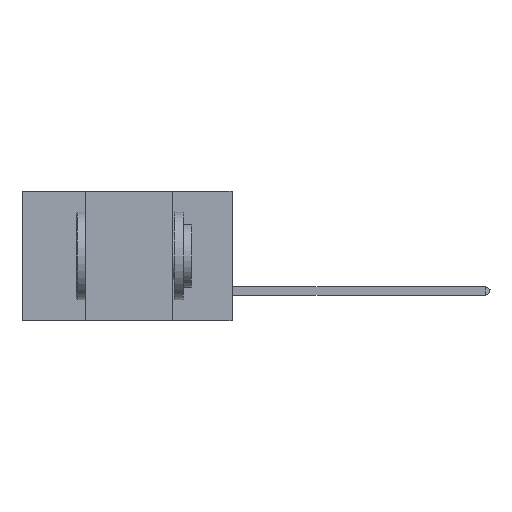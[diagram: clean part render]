
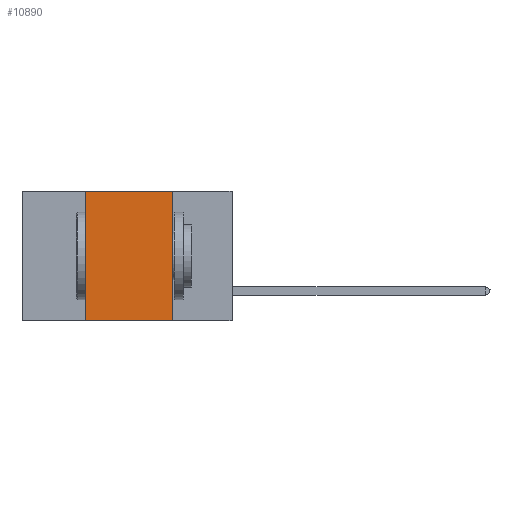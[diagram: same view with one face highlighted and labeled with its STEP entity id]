
A CAD part, left-side view. The second image highlights one B-rep face of the part: STEP entity #10890.
In plain terms, the highlighted planar face has unit normal (-1, 0, 0).
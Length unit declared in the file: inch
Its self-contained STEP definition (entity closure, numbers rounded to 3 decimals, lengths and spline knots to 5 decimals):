
#165 = DIRECTION ( 'NONE',  ( 0., 0., 1. ) ) ;
#483 = AXIS2_PLACEMENT_3D ( 'NONE', #10939, #2225, #4361 ) ;
#484 = CARTESIAN_POINT ( 'NONE',  ( 0., 0.6, -0.37 ) ) ;
#1360 = VERTEX_POINT ( 'NONE', #13789 ) ;
#1533 = VERTEX_POINT ( 'NONE', #3362 ) ;
#1584 = EDGE_LOOP ( 'NONE', ( #12478, #13533, #6326, #3112 ) ) ;
#1849 = VERTEX_POINT ( 'NONE', #3999 ) ;
#1929 = DIRECTION ( 'NONE',  ( 0., 0., -1. ) ) ;
#2007 = CARTESIAN_POINT ( 'NONE',  ( 0., 0.42, 0. ) ) ;
#2194 = VECTOR ( 'NONE', #11205, 39.37008 ) ;
#2225 = DIRECTION ( 'NONE',  ( 1., 0., 0. ) ) ;
#2637 = FACE_OUTER_BOUND ( 'NONE', #1584, .T. ) ;
#2908 = CARTESIAN_POINT ( 'NONE',  ( 0., 0.17, 0. ) ) ;
#2979 = LINE ( 'NONE', #9774, #13731 ) ;
#3112 = ORIENTED_EDGE ( 'NONE', *, *, #5513, .T. ) ;
#3362 = CARTESIAN_POINT ( 'NONE',  ( 0., 0.17, 0. ) ) ;
#3999 = CARTESIAN_POINT ( 'NONE',  ( 0., 0.42, -0.37 ) ) ;
#4361 = DIRECTION ( 'NONE',  ( 0., 0., -1. ) ) ;
#4731 = VERTEX_POINT ( 'NONE', #2007 ) ;
#5513 = EDGE_CURVE ( 'NONE', #1849, #1360, #10258, .T. ) ;
#6317 = VECTOR ( 'NONE', #1929, 39.37008 ) ;
#6326 = ORIENTED_EDGE ( 'NONE', *, *, #7049, .F. ) ;
#6571 = PLANE ( 'NONE',  #483 ) ;
#7049 = EDGE_CURVE ( 'NONE', #1849, #4731, #2979, .T. ) ;
#8129 = EDGE_CURVE ( 'NONE', #4731, #1533, #12055, .T. ) ;
#9686 = VECTOR ( 'NONE', #10607, 39.37008 ) ;
#9774 = CARTESIAN_POINT ( 'NONE',  ( 0., 0.42, 0. ) ) ;
#9877 = LINE ( 'NONE', #2908, #6317 ) ;
#10089 = EDGE_CURVE ( 'NONE', #1533, #1360, #9877, .T. ) ;
#10258 = LINE ( 'NONE', #484, #2194 ) ;
#10568 = CARTESIAN_POINT ( 'NONE',  ( 0., 0.6, 0. ) ) ;
#10607 = DIRECTION ( 'NONE',  ( 0., -1., 0. ) ) ;
#10890 = ADVANCED_FACE ( 'NONE', ( #2637 ), #6571, .F. ) ;
#10939 = CARTESIAN_POINT ( 'NONE',  ( 0., 0.6, 0. ) ) ;
#11205 = DIRECTION ( 'NONE',  ( 0., -1., 0. ) ) ;
#12055 = LINE ( 'NONE', #10568, #9686 ) ;
#12478 = ORIENTED_EDGE ( 'NONE', *, *, #10089, .F. ) ;
#13533 = ORIENTED_EDGE ( 'NONE', *, *, #8129, .F. ) ;
#13731 = VECTOR ( 'NONE', #165, 39.37008 ) ;
#13789 = CARTESIAN_POINT ( 'NONE',  ( 0., 0.17, -0.37 ) ) ;
